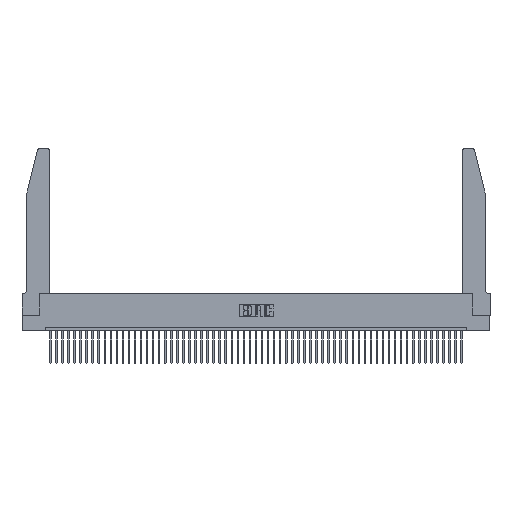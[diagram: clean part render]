
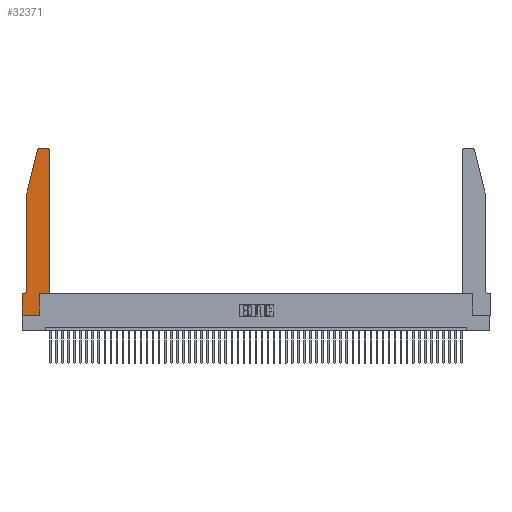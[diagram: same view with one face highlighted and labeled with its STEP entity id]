
A CAD part, top view. The second image highlights one B-rep face of the part: STEP entity #32371.
In plain terms, the highlighted planar face has unit normal (0, 0, 1).
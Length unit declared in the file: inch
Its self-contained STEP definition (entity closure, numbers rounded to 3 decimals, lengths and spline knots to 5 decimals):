
#391 = DIRECTION ( 'NONE',  ( 0., -1., 0. ) ) ;
#1210 = CARTESIAN_POINT ( 'NONE',  ( 0.0755, 0.35, 0.37 ) ) ;
#2534 = CARTESIAN_POINT ( 'NONE',  ( 0., 0., 0.37 ) ) ;
#2690 = CARTESIAN_POINT ( 'NONE',  ( 0.284, 2.72, 0.37 ) ) ;
#3080 = VERTEX_POINT ( 'NONE', #8188 ) ;
#3226 = CIRCLE ( 'NONE', #28514, 0.03 ) ;
#3300 = VECTOR ( 'NONE', #391, 39.37008 ) ;
#3477 = VECTOR ( 'NONE', #6296, 39.37008 ) ;
#3599 = CARTESIAN_POINT ( 'NONE',  ( 0., 0., 0.37 ) ) ;
#3936 = ORIENTED_EDGE ( 'NONE', *, *, #34371, .T. ) ;
#3950 = CARTESIAN_POINT ( 'NONE',  ( 0., 0., 0.37 ) ) ;
#4003 = PLANE ( 'NONE',  #26218 ) ;
#4362 = DIRECTION ( 'NONE',  ( 1., 0., 0. ) ) ;
#4434 = LINE ( 'NONE', #2534, #24852 ) ;
#5389 = DIRECTION ( 'NONE',  ( 0., 0., -1. ) ) ;
#6076 = LINE ( 'NONE', #6494, #38469 ) ;
#6296 = DIRECTION ( 'NONE',  ( 1., 0., 0. ) ) ;
#6494 = CARTESIAN_POINT ( 'NONE',  ( 0.2605, 2.75, 0.37 ) ) ;
#6597 = ORIENTED_EDGE ( 'NONE', *, *, #18179, .T. ) ;
#6812 = CARTESIAN_POINT ( 'NONE',  ( 0.2865, 0., 0.37 ) ) ;
#7518 = VECTOR ( 'NONE', #45864, 39.37008 ) ;
#8188 = CARTESIAN_POINT ( 'NONE',  ( 0.284, 2.75, 0.37 ) ) ;
#8668 = ORIENTED_EDGE ( 'NONE', *, *, #17811, .T. ) ;
#12432 = ORIENTED_EDGE ( 'NONE', *, *, #14888, .T. ) ;
#12965 = VERTEX_POINT ( 'NONE', #32099 ) ;
#13122 = VECTOR ( 'NONE', #25386, 39.37008 ) ;
#13668 = LINE ( 'NONE', #51450, #3477 ) ;
#13936 = LINE ( 'NONE', #17159, #7518 ) ;
#14032 = VERTEX_POINT ( 'NONE', #37749 ) ;
#14888 = EDGE_CURVE ( 'NONE', #40183, #40273, #43001, .T. ) ;
#15628 = EDGE_CURVE ( 'NONE', #3080, #45312, #3226, .T. ) ;
#16046 = DIRECTION ( 'NONE',  ( 1., 0., 0. ) ) ;
#16222 = CARTESIAN_POINT ( 'NONE',  ( 0.4205, 2.72, 0.37 ) ) ;
#16379 = DIRECTION ( 'NONE',  ( -0.239, -0.971, 0. ) ) ;
#16474 = EDGE_CURVE ( 'NONE', #18651, #40183, #29299, .T. ) ;
#16771 = AXIS2_PLACEMENT_3D ( 'NONE', #25756, #5389, #34682 ) ;
#17159 = CARTESIAN_POINT ( 'NONE',  ( 0.0755, 2., 0.37 ) ) ;
#17359 = CARTESIAN_POINT ( 'NONE',  ( 0.4505, 0.35, 0.37 ) ) ;
#17620 = DIRECTION ( 'NONE',  ( -1., 0., 0. ) ) ;
#17811 = EDGE_CURVE ( 'NONE', #40273, #3080, #6076, .T. ) ;
#18179 = EDGE_CURVE ( 'NONE', #12965, #18354, #13936, .T. ) ;
#18354 = VERTEX_POINT ( 'NONE', #26744 ) ;
#18651 = VERTEX_POINT ( 'NONE', #28364 ) ;
#18855 = DIRECTION ( 'NONE',  ( -1., 0., 0. ) ) ;
#19390 = VERTEX_POINT ( 'NONE', #3599 ) ;
#23212 = DIRECTION ( 'NONE',  ( 1., 0., 0. ) ) ;
#23350 = CARTESIAN_POINT ( 'NONE',  ( 0.25487, 2.72718, 0.37 ) ) ;
#24852 = VECTOR ( 'NONE', #23212, 39.37008 ) ;
#24969 = EDGE_CURVE ( 'NONE', #18354, #35803, #38006, .T. ) ;
#25008 = CARTESIAN_POINT ( 'NONE',  ( 0.4505, 2.72, 0.37 ) ) ;
#25386 = DIRECTION ( 'NONE',  ( 0., 1., 0. ) ) ;
#25756 = CARTESIAN_POINT ( 'NONE',  ( 0.0055, 0.42, 0.37 ) ) ;
#25923 = EDGE_LOOP ( 'NONE', ( #8668, #32317, #31965, #6597, #46116, #49728, #36840, #43124, #49783, #3936, #38063, #12432 ) ) ;
#26218 = AXIS2_PLACEMENT_3D ( 'NONE', #36518, #28832, #4362 ) ;
#26553 = EDGE_CURVE ( 'NONE', #35803, #27232, #44327, .T. ) ;
#26744 = CARTESIAN_POINT ( 'NONE',  ( 0.0755, 0.42, 0.37 ) ) ;
#27061 = CARTESIAN_POINT ( 'NONE',  ( 0.0055, 0.35, 0.37 ) ) ;
#27232 = VERTEX_POINT ( 'NONE', #43092 ) ;
#27981 = CARTESIAN_POINT ( 'NONE',  ( 0.0755, 2., 0.37 ) ) ;
#28364 = CARTESIAN_POINT ( 'NONE',  ( 0.4505, 0.35, 0.37 ) ) ;
#28365 = EDGE_CURVE ( 'NONE', #45312, #12965, #35122, .T. ) ;
#28514 = AXIS2_PLACEMENT_3D ( 'NONE', #2690, #39484, #16046 ) ;
#28555 = DIRECTION ( 'NONE',  ( 0., 0., 1. ) ) ;
#28832 = DIRECTION ( 'NONE',  ( 0., 0., 1. ) ) ;
#29120 = LINE ( 'NONE', #45719, #13122 ) ;
#29299 = LINE ( 'NONE', #17359, #33754 ) ;
#30861 = AXIS2_PLACEMENT_3D ( 'NONE', #16222, #28555, #32831 ) ;
#30949 = EDGE_CURVE ( 'NONE', #19390, #37735, #4434, .T. ) ;
#31149 = FACE_OUTER_BOUND ( 'NONE', #25923, .T. ) ;
#31965 = ORIENTED_EDGE ( 'NONE', *, *, #28365, .T. ) ;
#32099 = CARTESIAN_POINT ( 'NONE',  ( 0.0755, 2., 0.37 ) ) ;
#32317 = ORIENTED_EDGE ( 'NONE', *, *, #15628, .T. ) ;
#32371 = ADVANCED_FACE ( 'NONE', ( #31149 ), #4003, .T. ) ;
#32571 = VECTOR ( 'NONE', #16379, 39.37008 ) ;
#32831 = DIRECTION ( 'NONE',  ( 1., 0., 0. ) ) ;
#33754 = VECTOR ( 'NONE', #50147, 39.37008 ) ;
#34371 = EDGE_CURVE ( 'NONE', #14032, #18651, #13668, .T. ) ;
#34682 = DIRECTION ( 'NONE',  ( -1., 0., 0. ) ) ;
#35122 = LINE ( 'NONE', #27981, #32571 ) ;
#35803 = VERTEX_POINT ( 'NONE', #27061 ) ;
#35951 = VECTOR ( 'NONE', #17620, 39.37008 ) ;
#36518 = CARTESIAN_POINT ( 'NONE',  ( 0., 0.35, 0.37 ) ) ;
#36840 = ORIENTED_EDGE ( 'NONE', *, *, #38777, .T. ) ;
#37735 = VERTEX_POINT ( 'NONE', #6812 ) ;
#37749 = CARTESIAN_POINT ( 'NONE',  ( 0.2865, 0.35, 0.37 ) ) ;
#38006 = CIRCLE ( 'NONE', #16771, 0.07 ) ;
#38063 = ORIENTED_EDGE ( 'NONE', *, *, #16474, .T. ) ;
#38469 = VECTOR ( 'NONE', #18855, 39.37008 ) ;
#38777 = EDGE_CURVE ( 'NONE', #27232, #19390, #52000, .T. ) ;
#39484 = DIRECTION ( 'NONE',  ( 0., 0., 1. ) ) ;
#40183 = VERTEX_POINT ( 'NONE', #25008 ) ;
#40273 = VERTEX_POINT ( 'NONE', #51663 ) ;
#42660 = EDGE_CURVE ( 'NONE', #37735, #14032, #29120, .T. ) ;
#43001 = CIRCLE ( 'NONE', #30861, 0.03 ) ;
#43092 = CARTESIAN_POINT ( 'NONE',  ( 0., 0.35, 0.37 ) ) ;
#43124 = ORIENTED_EDGE ( 'NONE', *, *, #30949, .T. ) ;
#44327 = LINE ( 'NONE', #1210, #35951 ) ;
#45312 = VERTEX_POINT ( 'NONE', #23350 ) ;
#45719 = CARTESIAN_POINT ( 'NONE',  ( 0.2865, 0.35, 0.37 ) ) ;
#45864 = DIRECTION ( 'NONE',  ( 0., -1., 0. ) ) ;
#46116 = ORIENTED_EDGE ( 'NONE', *, *, #24969, .T. ) ;
#49728 = ORIENTED_EDGE ( 'NONE', *, *, #26553, .T. ) ;
#49783 = ORIENTED_EDGE ( 'NONE', *, *, #42660, .T. ) ;
#50147 = DIRECTION ( 'NONE',  ( 0., 1., 0. ) ) ;
#51450 = CARTESIAN_POINT ( 'NONE',  ( 0.4505, 0.35, 0.37 ) ) ;
#51663 = CARTESIAN_POINT ( 'NONE',  ( 0.4205, 2.75, 0.37 ) ) ;
#52000 = LINE ( 'NONE', #3950, #3300 ) ;
